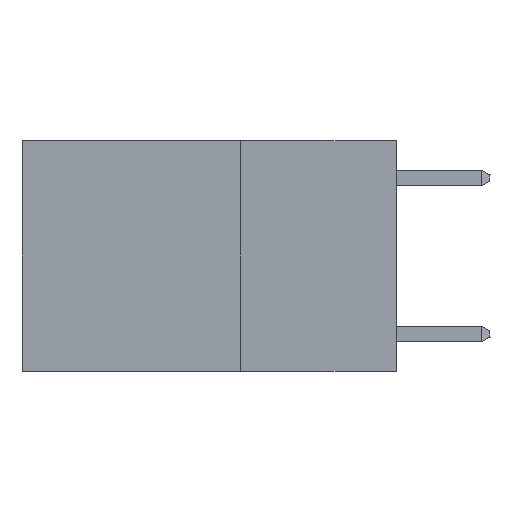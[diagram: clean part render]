
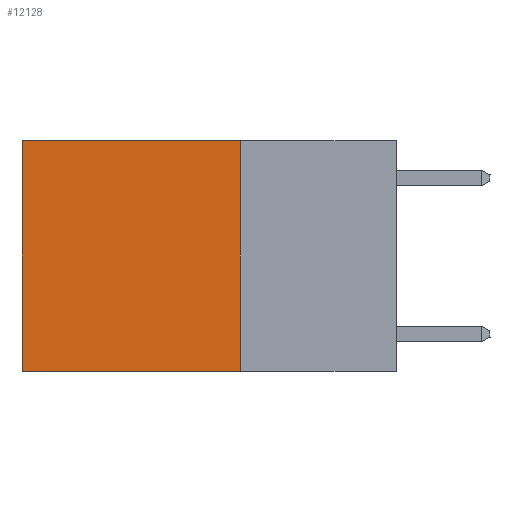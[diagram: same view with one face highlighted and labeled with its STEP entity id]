
A CAD part, left-side view. The second image highlights one B-rep face of the part: STEP entity #12128.
In plain terms, the highlighted planar face has unit normal (-1, 0, 0).
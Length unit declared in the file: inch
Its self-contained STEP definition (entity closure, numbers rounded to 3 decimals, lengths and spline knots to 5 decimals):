
#417 = CARTESIAN_POINT ( 'NONE',  ( 0.2625, 0.25, -0.37 ) ) ;
#550 = LINE ( 'NONE', #4229, #4491 ) ;
#1248 = VERTEX_POINT ( 'NONE', #6021 ) ;
#1448 = DIRECTION ( 'NONE',  ( 0., 0., -1. ) ) ;
#3185 = VECTOR ( 'NONE', #19599, 39.37008 ) ;
#4084 = DIRECTION ( 'NONE',  ( 0., 0., -1. ) ) ;
#4229 = CARTESIAN_POINT ( 'NONE',  ( 0.2625, 0.6, 0. ) ) ;
#4491 = VECTOR ( 'NONE', #19183, 39.37008 ) ;
#4967 = CARTESIAN_POINT ( 'NONE',  ( 0.2625, 0.6, 0. ) ) ;
#6021 = CARTESIAN_POINT ( 'NONE',  ( 0.2625, 0.25, 0. ) ) ;
#7028 = CARTESIAN_POINT ( 'NONE',  ( 0.2625, 0.25, -0.37 ) ) ;
#7086 = PLANE ( 'NONE',  #17303 ) ;
#8054 = VECTOR ( 'NONE', #4084, 39.37008 ) ;
#9019 = LINE ( 'NONE', #417, #17583 ) ;
#9324 = CARTESIAN_POINT ( 'NONE',  ( 0.2625, 0.25, 0. ) ) ;
#9589 = ORIENTED_EDGE ( 'NONE', *, *, #19264, .F. ) ;
#10390 = DIRECTION ( 'NONE',  ( 1., 0., 0. ) ) ;
#12076 = EDGE_CURVE ( 'NONE', #1248, #17313, #12114, .T. ) ;
#12114 = LINE ( 'NONE', #17528, #3185 ) ;
#12128 = ADVANCED_FACE ( 'NONE', ( #16158 ), #7086, .F. ) ;
#13085 = EDGE_LOOP ( 'NONE', ( #23602, #21653, #9589, #13212 ) ) ;
#13212 = ORIENTED_EDGE ( 'NONE', *, *, #12076, .T. ) ;
#13406 = LINE ( 'NONE', #9324, #8054 ) ;
#14534 = VERTEX_POINT ( 'NONE', #7028 ) ;
#15765 = VERTEX_POINT ( 'NONE', #21885 ) ;
#16158 = FACE_OUTER_BOUND ( 'NONE', #13085, .T. ) ;
#17303 = AXIS2_PLACEMENT_3D ( 'NONE', #23782, #10390, #1448 ) ;
#17313 = VERTEX_POINT ( 'NONE', #4967 ) ;
#17528 = CARTESIAN_POINT ( 'NONE',  ( 0.2625, 0.25, 0. ) ) ;
#17583 = VECTOR ( 'NONE', #20331, 39.37008 ) ;
#18949 = EDGE_CURVE ( 'NONE', #17313, #15765, #550, .T. ) ;
#19183 = DIRECTION ( 'NONE',  ( 0., 0., -1. ) ) ;
#19264 = EDGE_CURVE ( 'NONE', #1248, #14534, #13406, .T. ) ;
#19599 = DIRECTION ( 'NONE',  ( 0., 1., 0. ) ) ;
#20331 = DIRECTION ( 'NONE',  ( 0., 1., 0. ) ) ;
#21653 = ORIENTED_EDGE ( 'NONE', *, *, #22548, .F. ) ;
#21885 = CARTESIAN_POINT ( 'NONE',  ( 0.2625, 0.6, -0.37 ) ) ;
#22548 = EDGE_CURVE ( 'NONE', #14534, #15765, #9019, .T. ) ;
#23602 = ORIENTED_EDGE ( 'NONE', *, *, #18949, .T. ) ;
#23782 = CARTESIAN_POINT ( 'NONE',  ( 0.2625, 0.25, 0. ) ) ;
